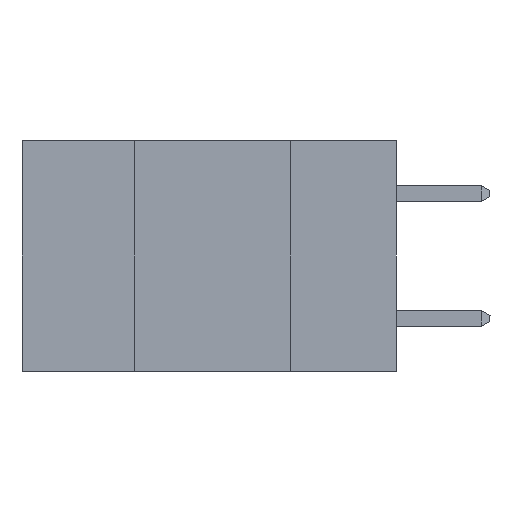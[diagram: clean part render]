
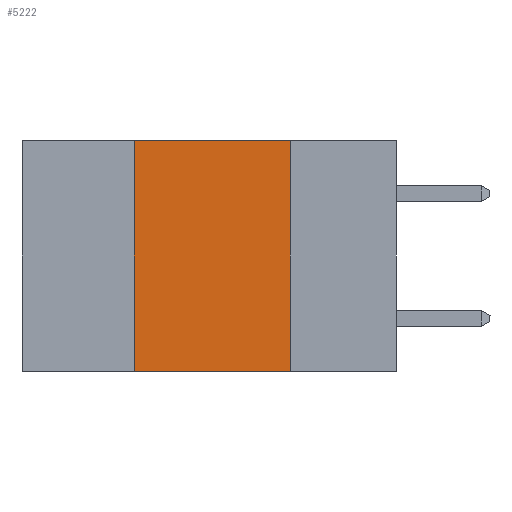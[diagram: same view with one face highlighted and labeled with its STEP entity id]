
A CAD part, left-side view. The second image highlights one B-rep face of the part: STEP entity #5222.
In plain terms, the highlighted planar face has unit normal (-1, 0, 0).
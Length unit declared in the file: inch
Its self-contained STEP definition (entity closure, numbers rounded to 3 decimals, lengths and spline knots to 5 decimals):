
#74 = VERTEX_POINT ( 'NONE', #1992 ) ;
#613 = CARTESIAN_POINT ( 'NONE',  ( 0., 0.17, 0. ) ) ;
#1130 = VERTEX_POINT ( 'NONE', #5614 ) ;
#1342 = FACE_OUTER_BOUND ( 'NONE', #20449, .T. ) ;
#1480 = EDGE_CURVE ( 'NONE', #1130, #7385, #14125, .T. ) ;
#1842 = CARTESIAN_POINT ( 'NONE',  ( 0., 0.6, 0. ) ) ;
#1992 = CARTESIAN_POINT ( 'NONE',  ( 0., 0.17, -0.37 ) ) ;
#2011 = DIRECTION ( 'NONE',  ( 1., 0., 0. ) ) ;
#3441 = CARTESIAN_POINT ( 'NONE',  ( 0., 0.42, 0. ) ) ;
#3988 = EDGE_CURVE ( 'NONE', #7385, #17859, #15234, .T. ) ;
#5222 = ADVANCED_FACE ( 'NONE', ( #1342 ), #9792, .F. ) ;
#5614 = CARTESIAN_POINT ( 'NONE',  ( 0., 0.42, -0.37 ) ) ;
#6153 = DIRECTION ( 'NONE',  ( 0., 0., -1. ) ) ;
#7385 = VERTEX_POINT ( 'NONE', #11305 ) ;
#8466 = VECTOR ( 'NONE', #24825, 39.37008 ) ;
#9584 = CARTESIAN_POINT ( 'NONE',  ( 0., 0.6, -0.37 ) ) ;
#9792 = PLANE ( 'NONE',  #21727 ) ;
#11305 = CARTESIAN_POINT ( 'NONE',  ( 0., 0.42, 0. ) ) ;
#11866 = DIRECTION ( 'NONE',  ( 0., 0., 1. ) ) ;
#12155 = ORIENTED_EDGE ( 'NONE', *, *, #1480, .F. ) ;
#12430 = DIRECTION ( 'NONE',  ( 0., -1., 0. ) ) ;
#12644 = LINE ( 'NONE', #9584, #8466 ) ;
#14125 = LINE ( 'NONE', #3441, #20072 ) ;
#15234 = LINE ( 'NONE', #23747, #17623 ) ;
#16313 = EDGE_CURVE ( 'NONE', #17859, #74, #16695, .T. ) ;
#16419 = ORIENTED_EDGE ( 'NONE', *, *, #3988, .F. ) ;
#16695 = LINE ( 'NONE', #613, #24519 ) ;
#17287 = DIRECTION ( 'NONE',  ( 0., 0., -1. ) ) ;
#17623 = VECTOR ( 'NONE', #12430, 39.37008 ) ;
#17859 = VERTEX_POINT ( 'NONE', #23942 ) ;
#20072 = VECTOR ( 'NONE', #11866, 39.37008 ) ;
#20419 = ORIENTED_EDGE ( 'NONE', *, *, #16313, .F. ) ;
#20449 = EDGE_LOOP ( 'NONE', ( #20419, #16419, #12155, #22563 ) ) ;
#21727 = AXIS2_PLACEMENT_3D ( 'NONE', #1842, #2011, #17287 ) ;
#21752 = EDGE_CURVE ( 'NONE', #1130, #74, #12644, .T. ) ;
#22563 = ORIENTED_EDGE ( 'NONE', *, *, #21752, .T. ) ;
#23747 = CARTESIAN_POINT ( 'NONE',  ( 0., 0.6, 0. ) ) ;
#23942 = CARTESIAN_POINT ( 'NONE',  ( 0., 0.17, 0. ) ) ;
#24519 = VECTOR ( 'NONE', #6153, 39.37008 ) ;
#24825 = DIRECTION ( 'NONE',  ( 0., -1., 0. ) ) ;
